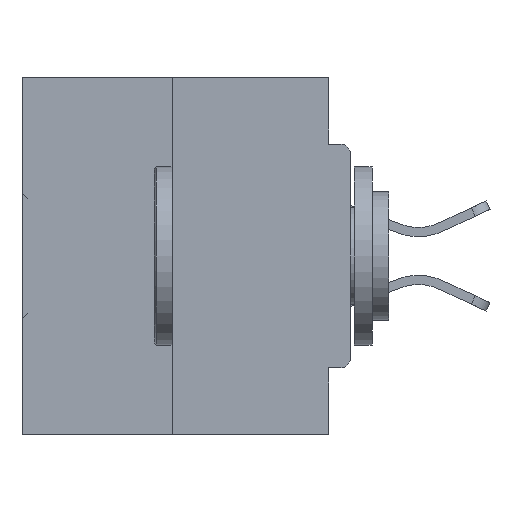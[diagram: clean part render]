
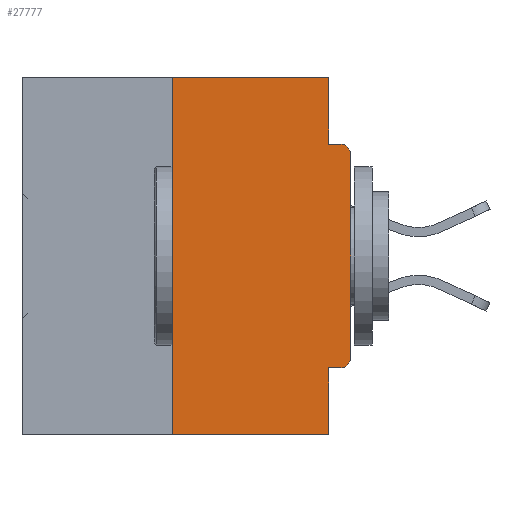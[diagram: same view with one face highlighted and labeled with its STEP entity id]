
A CAD part, left-side view. The second image highlights one B-rep face of the part: STEP entity #27777.
In plain terms, the highlighted planar face has unit normal (-1, 0, 0).
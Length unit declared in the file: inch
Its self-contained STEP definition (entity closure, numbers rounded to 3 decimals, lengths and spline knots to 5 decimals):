
#93 = CARTESIAN_POINT ( 'NONE',  ( 0., 0., -0.3915 ) ) ;
#111 = EDGE_CURVE ( 'NONE', #7407, #22213, #40318, .T. ) ;
#291 = CARTESIAN_POINT ( 'NONE',  ( 0., 0.031, -0.4065 ) ) ;
#335 = EDGE_CURVE ( 'NONE', #45939, #12912, #20066, .T. ) ;
#522 = VECTOR ( 'NONE', #25483, 39.37008 ) ;
#1339 = CARTESIAN_POINT ( 'NONE',  ( 0., 0.031, 0. ) ) ;
#1522 = ORIENTED_EDGE ( 'NONE', *, *, #16029, .F. ) ;
#2194 = EDGE_CURVE ( 'NONE', #44406, #18512, #15312, .T. ) ;
#4005 = ORIENTED_EDGE ( 'NONE', *, *, #19342, .T. ) ;
#6086 = LINE ( 'NONE', #6899, #34300 ) ;
#6560 = VERTEX_POINT ( 'NONE', #13542 ) ;
#6899 = CARTESIAN_POINT ( 'NONE',  ( 0., 0.46, -0.5 ) ) ;
#7407 = VERTEX_POINT ( 'NONE', #25569 ) ;
#7803 = DIRECTION ( 'NONE',  ( 0., 0., 1. ) ) ;
#9163 = CARTESIAN_POINT ( 'NONE',  ( 0., 0.015, -0.1085 ) ) ;
#9520 = EDGE_CURVE ( 'NONE', #30996, #44550, #6086, .T. ) ;
#12227 = EDGE_CURVE ( 'NONE', #30996, #7407, #24863, .T. ) ;
#12252 = DIRECTION ( 'NONE',  ( 0., 0., -1. ) ) ;
#12830 = CARTESIAN_POINT ( 'NONE',  ( 0., 0.25, 0. ) ) ;
#12912 = VERTEX_POINT ( 'NONE', #19429 ) ;
#13542 = CARTESIAN_POINT ( 'NONE',  ( 0., 0., -0.1085 ) ) ;
#13584 = EDGE_CURVE ( 'NONE', #18512, #6560, #24648, .T. ) ;
#13912 = CARTESIAN_POINT ( 'NONE',  ( 0., 0.015, -0.3915 ) ) ;
#15128 = CARTESIAN_POINT ( 'NONE',  ( 0., 0.031, -0.0935 ) ) ;
#15312 = CIRCLE ( 'NONE', #43737, 0.015 ) ;
#16029 = EDGE_CURVE ( 'NONE', #44406, #43216, #36048, .T. ) ;
#16537 = DIRECTION ( 'NONE',  ( 0., 0., 1. ) ) ;
#17239 = CARTESIAN_POINT ( 'NONE',  ( 0., 0.031, -0.5 ) ) ;
#17448 = CARTESIAN_POINT ( 'NONE',  ( 0., 0.46, 0. ) ) ;
#18491 = ORIENTED_EDGE ( 'NONE', *, *, #13584, .T. ) ;
#18512 = VERTEX_POINT ( 'NONE', #93 ) ;
#18777 = VECTOR ( 'NONE', #7803, 39.37008 ) ;
#19342 = EDGE_CURVE ( 'NONE', #6560, #12912, #29208, .T. ) ;
#19429 = CARTESIAN_POINT ( 'NONE',  ( 0., 0.015, -0.0935 ) ) ;
#20066 = LINE ( 'NONE', #36873, #522 ) ;
#20909 = CARTESIAN_POINT ( 'NONE',  ( 0., 0.031, 0. ) ) ;
#21116 = LINE ( 'NONE', #1339, #43066 ) ;
#21283 = DIRECTION ( 'NONE',  ( 0., 0., -1. ) ) ;
#21864 = VECTOR ( 'NONE', #28284, 39.37008 ) ;
#22213 = VERTEX_POINT ( 'NONE', #20909 ) ;
#22386 = AXIS2_PLACEMENT_3D ( 'NONE', #26523, #22976, #22506 ) ;
#22506 = DIRECTION ( 'NONE',  ( 0., 0., -1. ) ) ;
#22976 = DIRECTION ( 'NONE',  ( 1., 0., 0. ) ) ;
#24257 = VECTOR ( 'NONE', #16537, 39.37008 ) ;
#24648 = LINE ( 'NONE', #40325, #18777 ) ;
#24863 = LINE ( 'NONE', #12830, #24257 ) ;
#25180 = DIRECTION ( 'NONE',  ( -1., 0., 0. ) ) ;
#25341 = LINE ( 'NONE', #37724, #45456 ) ;
#25483 = DIRECTION ( 'NONE',  ( 0., -1., 0. ) ) ;
#25569 = CARTESIAN_POINT ( 'NONE',  ( 0., 0.25, 0. ) ) ;
#25836 = ORIENTED_EDGE ( 'NONE', *, *, #335, .F. ) ;
#26281 = VECTOR ( 'NONE', #39388, 39.37008 ) ;
#26523 = CARTESIAN_POINT ( 'NONE',  ( 0., 0.46, 0. ) ) ;
#27777 = ADVANCED_FACE ( 'NONE', ( #40730 ), #44897, .F. ) ;
#28284 = DIRECTION ( 'NONE',  ( 0., -1., 0. ) ) ;
#28653 = ORIENTED_EDGE ( 'NONE', *, *, #9520, .T. ) ;
#29208 = CIRCLE ( 'NONE', #29488, 0.015 ) ;
#29488 = AXIS2_PLACEMENT_3D ( 'NONE', #9163, #31008, #42157 ) ;
#29649 = ORIENTED_EDGE ( 'NONE', *, *, #111, .F. ) ;
#30603 = CARTESIAN_POINT ( 'NONE',  ( 0., 0.25, -0.5 ) ) ;
#30996 = VERTEX_POINT ( 'NONE', #30603 ) ;
#31008 = DIRECTION ( 'NONE',  ( -1., 0., 0. ) ) ;
#33121 = DIRECTION ( 'NONE',  ( 0., -1., 0. ) ) ;
#33902 = EDGE_CURVE ( 'NONE', #22213, #45939, #21116, .T. ) ;
#34300 = VECTOR ( 'NONE', #33121, 39.37008 ) ;
#36048 = LINE ( 'NONE', #36148, #26281 ) ;
#36148 = CARTESIAN_POINT ( 'NONE',  ( 0., 0., -0.4065 ) ) ;
#36873 = CARTESIAN_POINT ( 'NONE',  ( 0., 0., -0.0935 ) ) ;
#37410 = EDGE_CURVE ( 'NONE', #43216, #44550, #25341, .T. ) ;
#37724 = CARTESIAN_POINT ( 'NONE',  ( 0., 0.031, -0.5 ) ) ;
#39388 = DIRECTION ( 'NONE',  ( 0., 1., 0. ) ) ;
#39521 = ORIENTED_EDGE ( 'NONE', *, *, #2194, .T. ) ;
#39994 = ORIENTED_EDGE ( 'NONE', *, *, #37410, .F. ) ;
#40318 = LINE ( 'NONE', #17448, #21864 ) ;
#40325 = CARTESIAN_POINT ( 'NONE',  ( 0., 0., 0. ) ) ;
#40730 = FACE_OUTER_BOUND ( 'NONE', #43812, .T. ) ;
#41751 = CARTESIAN_POINT ( 'NONE',  ( 0., 0.015, -0.4065 ) ) ;
#42157 = DIRECTION ( 'NONE',  ( 0., 0., -1. ) ) ;
#43066 = VECTOR ( 'NONE', #12252, 39.37008 ) ;
#43216 = VERTEX_POINT ( 'NONE', #291 ) ;
#43737 = AXIS2_PLACEMENT_3D ( 'NONE', #13912, #25180, #21283 ) ;
#43812 = EDGE_LOOP ( 'NONE', ( #29649, #45550, #28653, #39994, #1522, #39521, #18491, #4005, #25836, #47513 ) ) ;
#44406 = VERTEX_POINT ( 'NONE', #41751 ) ;
#44550 = VERTEX_POINT ( 'NONE', #17239 ) ;
#44897 = PLANE ( 'NONE',  #22386 ) ;
#45456 = VECTOR ( 'NONE', #45610, 39.37008 ) ;
#45550 = ORIENTED_EDGE ( 'NONE', *, *, #12227, .F. ) ;
#45610 = DIRECTION ( 'NONE',  ( 0., 0., -1. ) ) ;
#45939 = VERTEX_POINT ( 'NONE', #15128 ) ;
#47513 = ORIENTED_EDGE ( 'NONE', *, *, #33902, .F. ) ;
